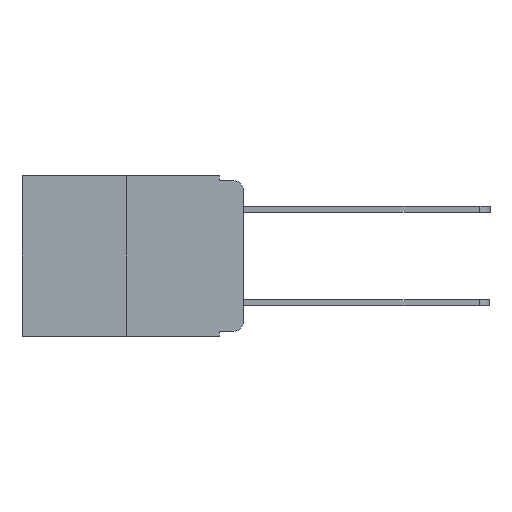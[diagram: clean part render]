
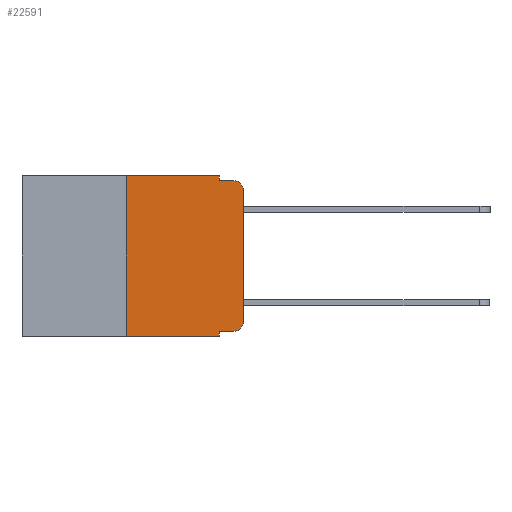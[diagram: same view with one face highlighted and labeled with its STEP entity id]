
A CAD part, left-side view. The second image highlights one B-rep face of the part: STEP entity #22591.
In plain terms, the highlighted planar face has unit normal (-1, 0, 0).
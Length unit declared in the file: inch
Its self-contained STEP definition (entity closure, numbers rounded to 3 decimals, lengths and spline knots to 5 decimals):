
#118 = ORIENTED_EDGE ( 'NONE', *, *, #13195, .T. ) ;
#937 = VERTEX_POINT ( 'NONE', #18085 ) ;
#1011 = ORIENTED_EDGE ( 'NONE', *, *, #15309, .F. ) ;
#1249 = CARTESIAN_POINT ( 'NONE',  ( 0., 0.473, 0. ) ) ;
#1760 = LINE ( 'NONE', #9019, #11225 ) ;
#2116 = FACE_OUTER_BOUND ( 'NONE', #9895, .T. ) ;
#2144 = VECTOR ( 'NONE', #17770, 39.37008 ) ;
#2167 = ORIENTED_EDGE ( 'NONE', *, *, #2426, .T. ) ;
#2426 = EDGE_CURVE ( 'NONE', #14641, #20726, #10575, .T. ) ;
#2985 = DIRECTION ( 'NONE',  ( -1., 0., 0. ) ) ;
#3443 = CARTESIAN_POINT ( 'NONE',  ( 0., 0.02, -0.01 ) ) ;
#3749 = CARTESIAN_POINT ( 'NONE',  ( 0., 0.051, 0. ) ) ;
#3774 = VECTOR ( 'NONE', #19646, 39.37008 ) ;
#4441 = EDGE_CURVE ( 'NONE', #7755, #5322, #17923, .T. ) ;
#5322 = VERTEX_POINT ( 'NONE', #3443 ) ;
#5410 = DIRECTION ( 'NONE',  ( -1., 0., 0. ) ) ;
#5437 = VECTOR ( 'NONE', #10066, 39.37008 ) ;
#6013 = LINE ( 'NONE', #15271, #5437 ) ;
#6638 = CIRCLE ( 'NONE', #22609, 0.02 ) ;
#6780 = DIRECTION ( 'NONE',  ( 0., -1., 0. ) ) ;
#6965 = DIRECTION ( 'NONE',  ( 0., 0., 1. ) ) ;
#7755 = VERTEX_POINT ( 'NONE', #12120 ) ;
#8120 = ORIENTED_EDGE ( 'NONE', *, *, #15203, .T. ) ;
#8390 = ORIENTED_EDGE ( 'NONE', *, *, #17258, .T. ) ;
#8535 = LINE ( 'NONE', #14467, #3774 ) ;
#8662 = VECTOR ( 'NONE', #18102, 39.37008 ) ;
#9019 = CARTESIAN_POINT ( 'NONE',  ( 0., 0.051, -0.333 ) ) ;
#9027 = CARTESIAN_POINT ( 'NONE',  ( 0., 0.473, -0.343 ) ) ;
#9842 = CARTESIAN_POINT ( 'NONE',  ( 0., 0.051, 0. ) ) ;
#9871 = EDGE_CURVE ( 'NONE', #19637, #7755, #21927, .T. ) ;
#9895 = EDGE_LOOP ( 'NONE', ( #16603, #8390, #12982, #22647, #1011, #20277, #2167, #16885, #8120, #118 ) ) ;
#10066 = DIRECTION ( 'NONE',  ( 0., 0., -1. ) ) ;
#10238 = DIRECTION ( 'NONE',  ( 0., 0., -1. ) ) ;
#10575 = LINE ( 'NONE', #9027, #18766 ) ;
#10727 = VERTEX_POINT ( 'NONE', #20688 ) ;
#11225 = VECTOR ( 'NONE', #17768, 39.37008 ) ;
#12103 = CARTESIAN_POINT ( 'NONE',  ( 0., 0.051, -0.333 ) ) ;
#12120 = CARTESIAN_POINT ( 'NONE',  ( 0., 0.051, -0.01 ) ) ;
#12982 = ORIENTED_EDGE ( 'NONE', *, *, #4441, .F. ) ;
#13149 = VERTEX_POINT ( 'NONE', #19134 ) ;
#13195 = EDGE_CURVE ( 'NONE', #937, #10727, #22122, .T. ) ;
#13569 = CARTESIAN_POINT ( 'NONE',  ( 0., 0.02, -0.03 ) ) ;
#13664 = LINE ( 'NONE', #15685, #22246 ) ;
#14064 = CARTESIAN_POINT ( 'NONE',  ( 0., 0.051, -0.01 ) ) ;
#14420 = CARTESIAN_POINT ( 'NONE',  ( 0., 0.25, -0.343 ) ) ;
#14467 = CARTESIAN_POINT ( 'NONE',  ( 0., 0.473, 0. ) ) ;
#14545 = AXIS2_PLACEMENT_3D ( 'NONE', #15921, #5410, #17669 ) ;
#14641 = VERTEX_POINT ( 'NONE', #14420 ) ;
#15203 = EDGE_CURVE ( 'NONE', #20139, #937, #1760, .T. ) ;
#15271 = CARTESIAN_POINT ( 'NONE',  ( 0., 0.051, 0. ) ) ;
#15309 = EDGE_CURVE ( 'NONE', #13149, #19637, #8535, .T. ) ;
#15338 = DIRECTION ( 'NONE',  ( 0., 0., -1. ) ) ;
#15685 = CARTESIAN_POINT ( 'NONE',  ( 0., 0., 0. ) ) ;
#15748 = EDGE_CURVE ( 'NONE', #10727, #16634, #13664, .T. ) ;
#15921 = CARTESIAN_POINT ( 'NONE',  ( 0., 0.02, -0.313 ) ) ;
#16603 = ORIENTED_EDGE ( 'NONE', *, *, #15748, .T. ) ;
#16634 = VERTEX_POINT ( 'NONE', #20374 ) ;
#16862 = LINE ( 'NONE', #21126, #2144 ) ;
#16885 = ORIENTED_EDGE ( 'NONE', *, *, #19013, .F. ) ;
#17258 = EDGE_CURVE ( 'NONE', #16634, #5322, #6638, .T. ) ;
#17468 = VECTOR ( 'NONE', #21897, 39.37008 ) ;
#17669 = DIRECTION ( 'NONE',  ( 0., 0., -1. ) ) ;
#17768 = DIRECTION ( 'NONE',  ( 0., -1., 0. ) ) ;
#17770 = DIRECTION ( 'NONE',  ( 0., 0., 1. ) ) ;
#17923 = LINE ( 'NONE', #14064, #8662 ) ;
#18085 = CARTESIAN_POINT ( 'NONE',  ( 0., 0.02, -0.333 ) ) ;
#18102 = DIRECTION ( 'NONE',  ( 0., -1., 0. ) ) ;
#18350 = AXIS2_PLACEMENT_3D ( 'NONE', #1249, #20596, #10238 ) ;
#18766 = VECTOR ( 'NONE', #6780, 39.37008 ) ;
#18922 = PLANE ( 'NONE',  #18350 ) ;
#19013 = EDGE_CURVE ( 'NONE', #20139, #20726, #6013, .T. ) ;
#19134 = CARTESIAN_POINT ( 'NONE',  ( 0., 0.25, 0. ) ) ;
#19637 = VERTEX_POINT ( 'NONE', #3749 ) ;
#19646 = DIRECTION ( 'NONE',  ( 0., -1., 0. ) ) ;
#20139 = VERTEX_POINT ( 'NONE', #12103 ) ;
#20277 = ORIENTED_EDGE ( 'NONE', *, *, #22157, .F. ) ;
#20374 = CARTESIAN_POINT ( 'NONE',  ( 0., 0., -0.03 ) ) ;
#20596 = DIRECTION ( 'NONE',  ( 1., 0., 0. ) ) ;
#20688 = CARTESIAN_POINT ( 'NONE',  ( 0., 0., -0.313 ) ) ;
#20726 = VERTEX_POINT ( 'NONE', #22176 ) ;
#21126 = CARTESIAN_POINT ( 'NONE',  ( 0., 0.25, 0. ) ) ;
#21897 = DIRECTION ( 'NONE',  ( 0., 0., -1. ) ) ;
#21927 = LINE ( 'NONE', #9842, #17468 ) ;
#22122 = CIRCLE ( 'NONE', #14545, 0.02 ) ;
#22157 = EDGE_CURVE ( 'NONE', #14641, #13149, #16862, .T. ) ;
#22176 = CARTESIAN_POINT ( 'NONE',  ( 0., 0.051, -0.343 ) ) ;
#22246 = VECTOR ( 'NONE', #6965, 39.37008 ) ;
#22591 = ADVANCED_FACE ( 'NONE', ( #2116 ), #18922, .F. ) ;
#22609 = AXIS2_PLACEMENT_3D ( 'NONE', #13569, #2985, #15338 ) ;
#22647 = ORIENTED_EDGE ( 'NONE', *, *, #9871, .F. ) ;
